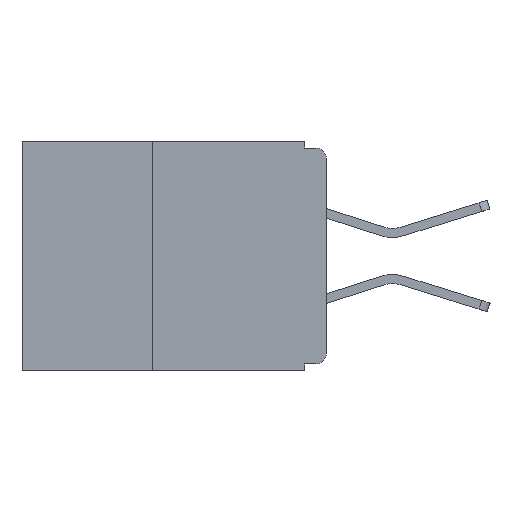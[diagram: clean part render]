
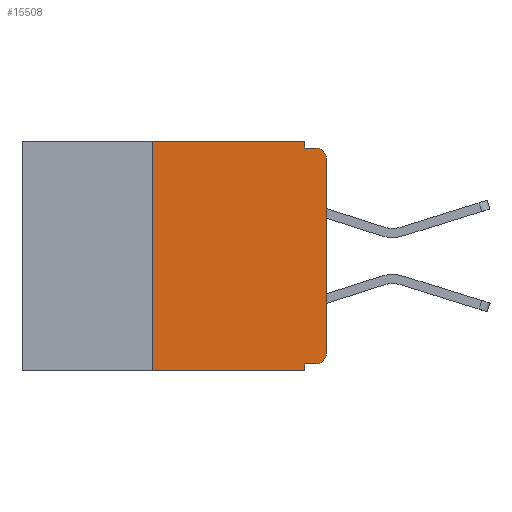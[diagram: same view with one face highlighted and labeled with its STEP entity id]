
A CAD part, left-side view. The second image highlights one B-rep face of the part: STEP entity #15508.
In plain terms, the highlighted planar face has unit normal (-1, 0, 0).
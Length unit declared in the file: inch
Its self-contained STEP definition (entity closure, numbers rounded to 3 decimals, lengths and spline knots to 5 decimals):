
#115 = EDGE_CURVE ( 'NONE', #1591, #16286, #9153, .T. ) ;
#209 = CARTESIAN_POINT ( 'NONE',  ( 0., 0.015, -0.32 ) ) ;
#424 = CARTESIAN_POINT ( 'NONE',  ( 0., 0.031, -0.33 ) ) ;
#483 = CARTESIAN_POINT ( 'NONE',  ( 0., 0., -0.025 ) ) ;
#802 = AXIS2_PLACEMENT_3D ( 'NONE', #5198, #14758, #6603 ) ;
#1359 = VERTEX_POINT ( 'NONE', #13717 ) ;
#1591 = VERTEX_POINT ( 'NONE', #7417 ) ;
#1711 = VERTEX_POINT ( 'NONE', #209 ) ;
#1923 = FACE_OUTER_BOUND ( 'NONE', #9020, .T. ) ;
#2040 = CARTESIAN_POINT ( 'NONE',  ( 0., 0.437, 0. ) ) ;
#2363 = CARTESIAN_POINT ( 'NONE',  ( 0., 0.437, 0. ) ) ;
#2419 = CARTESIAN_POINT ( 'NONE',  ( 0., 0., -0.01 ) ) ;
#2945 = VECTOR ( 'NONE', #6840, 39.37008 ) ;
#3077 = VERTEX_POINT ( 'NONE', #12165 ) ;
#3258 = CARTESIAN_POINT ( 'NONE',  ( 0., 0., -0.305 ) ) ;
#3365 = ORIENTED_EDGE ( 'NONE', *, *, #7562, .F. ) ;
#3396 = CARTESIAN_POINT ( 'NONE',  ( 0., 0.031, 0. ) ) ;
#3660 = VERTEX_POINT ( 'NONE', #9044 ) ;
#3723 = DIRECTION ( 'NONE',  ( 0., 0., -1. ) ) ;
#3779 = CARTESIAN_POINT ( 'NONE',  ( 0., 0.437, -0.33 ) ) ;
#4664 = EDGE_CURVE ( 'NONE', #1711, #3077, #7020, .T. ) ;
#4700 = VECTOR ( 'NONE', #13364, 39.37008 ) ;
#4919 = EDGE_CURVE ( 'NONE', #1711, #5674, #12791, .T. ) ;
#5198 = CARTESIAN_POINT ( 'NONE',  ( 0., 0.015, -0.025 ) ) ;
#5264 = VERTEX_POINT ( 'NONE', #9231 ) ;
#5366 = LINE ( 'NONE', #3396, #12266 ) ;
#5484 = VECTOR ( 'NONE', #12897, 39.37008 ) ;
#5674 = VERTEX_POINT ( 'NONE', #3258 ) ;
#5911 = LINE ( 'NONE', #424, #9559 ) ;
#6166 = ORIENTED_EDGE ( 'NONE', *, *, #14063, .T. ) ;
#6597 = ORIENTED_EDGE ( 'NONE', *, *, #12656, .F. ) ;
#6603 = DIRECTION ( 'NONE',  ( 0., 0., -1. ) ) ;
#6840 = DIRECTION ( 'NONE',  ( 0., 0., 1. ) ) ;
#7020 = LINE ( 'NONE', #8693, #16136 ) ;
#7079 = CARTESIAN_POINT ( 'NONE',  ( 0., 0., 0. ) ) ;
#7417 = CARTESIAN_POINT ( 'NONE',  ( 0., 0.25, 0. ) ) ;
#7457 = ORIENTED_EDGE ( 'NONE', *, *, #4664, .F. ) ;
#7471 = DIRECTION ( 'NONE',  ( 0., 1., 0. ) ) ;
#7562 = EDGE_CURVE ( 'NONE', #3660, #1591, #11595, .T. ) ;
#8099 = CARTESIAN_POINT ( 'NONE',  ( 0., 0.015, -0.01 ) ) ;
#8347 = VECTOR ( 'NONE', #16130, 39.37008 ) ;
#8413 = VERTEX_POINT ( 'NONE', #8099 ) ;
#8540 = EDGE_CURVE ( 'NONE', #5674, #13784, #13848, .T. ) ;
#8693 = CARTESIAN_POINT ( 'NONE',  ( 0., 0., -0.32 ) ) ;
#9020 = EDGE_LOOP ( 'NONE', ( #16544, #6166, #16941, #6597, #10252, #3365, #10682, #14276, #7457, #11118 ) ) ;
#9044 = CARTESIAN_POINT ( 'NONE',  ( 0., 0.25, -0.33 ) ) ;
#9153 = LINE ( 'NONE', #2040, #5484 ) ;
#9231 = CARTESIAN_POINT ( 'NONE',  ( 0., 0.031, -0.01 ) ) ;
#9559 = VECTOR ( 'NONE', #10040, 39.37008 ) ;
#9796 = LINE ( 'NONE', #2419, #13000 ) ;
#10040 = DIRECTION ( 'NONE',  ( 0., 0., -1. ) ) ;
#10252 = ORIENTED_EDGE ( 'NONE', *, *, #115, .F. ) ;
#10260 = DIRECTION ( 'NONE',  ( 0., 0., -1. ) ) ;
#10682 = ORIENTED_EDGE ( 'NONE', *, *, #15543, .T. ) ;
#11118 = ORIENTED_EDGE ( 'NONE', *, *, #4919, .T. ) ;
#11595 = LINE ( 'NONE', #16018, #8347 ) ;
#11976 = DIRECTION ( 'NONE',  ( 1., 0., 0. ) ) ;
#12165 = CARTESIAN_POINT ( 'NONE',  ( 0., 0.031, -0.32 ) ) ;
#12266 = VECTOR ( 'NONE', #10260, 39.37008 ) ;
#12656 = EDGE_CURVE ( 'NONE', #16286, #5264, #5366, .T. ) ;
#12791 = CIRCLE ( 'NONE', #14308, 0.015 ) ;
#12897 = DIRECTION ( 'NONE',  ( 0., -1., 0. ) ) ;
#13000 = VECTOR ( 'NONE', #14772, 39.37008 ) ;
#13364 = DIRECTION ( 'NONE',  ( 0., -1., 0. ) ) ;
#13625 = CARTESIAN_POINT ( 'NONE',  ( 0., 0.031, 0. ) ) ;
#13717 = CARTESIAN_POINT ( 'NONE',  ( 0., 0.031, -0.33 ) ) ;
#13784 = VERTEX_POINT ( 'NONE', #483 ) ;
#13848 = LINE ( 'NONE', #7079, #2945 ) ;
#14063 = EDGE_CURVE ( 'NONE', #13784, #8413, #15195, .T. ) ;
#14276 = ORIENTED_EDGE ( 'NONE', *, *, #17590, .F. ) ;
#14308 = AXIS2_PLACEMENT_3D ( 'NONE', #15366, #15341, #15303 ) ;
#14758 = DIRECTION ( 'NONE',  ( -1., 0., 0. ) ) ;
#14772 = DIRECTION ( 'NONE',  ( 0., -1., 0. ) ) ;
#15195 = CIRCLE ( 'NONE', #802, 0.015 ) ;
#15303 = DIRECTION ( 'NONE',  ( 0., 0., -1. ) ) ;
#15341 = DIRECTION ( 'NONE',  ( -1., 0., 0. ) ) ;
#15366 = CARTESIAN_POINT ( 'NONE',  ( 0., 0.015, -0.305 ) ) ;
#15508 = ADVANCED_FACE ( 'NONE', ( #1923 ), #15938, .F. ) ;
#15543 = EDGE_CURVE ( 'NONE', #3660, #1359, #15589, .T. ) ;
#15589 = LINE ( 'NONE', #3779, #4700 ) ;
#15899 = AXIS2_PLACEMENT_3D ( 'NONE', #2363, #11976, #3723 ) ;
#15938 = PLANE ( 'NONE',  #15899 ) ;
#16018 = CARTESIAN_POINT ( 'NONE',  ( 0., 0.25, -0.33 ) ) ;
#16130 = DIRECTION ( 'NONE',  ( 0., 0., 1. ) ) ;
#16136 = VECTOR ( 'NONE', #7471, 39.37008 ) ;
#16286 = VERTEX_POINT ( 'NONE', #13625 ) ;
#16544 = ORIENTED_EDGE ( 'NONE', *, *, #8540, .T. ) ;
#16941 = ORIENTED_EDGE ( 'NONE', *, *, #17342, .F. ) ;
#17342 = EDGE_CURVE ( 'NONE', #5264, #8413, #9796, .T. ) ;
#17590 = EDGE_CURVE ( 'NONE', #3077, #1359, #5911, .T. ) ;
